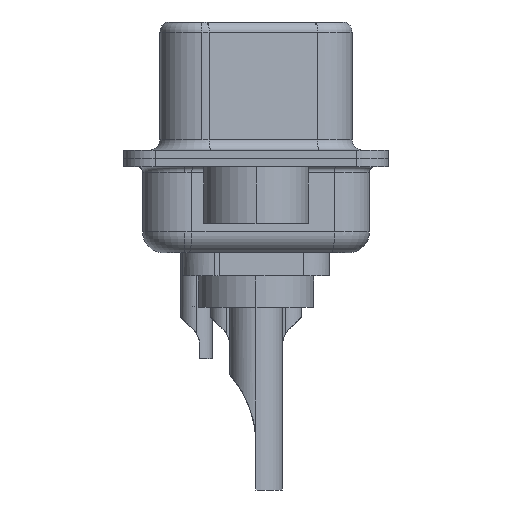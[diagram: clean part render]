
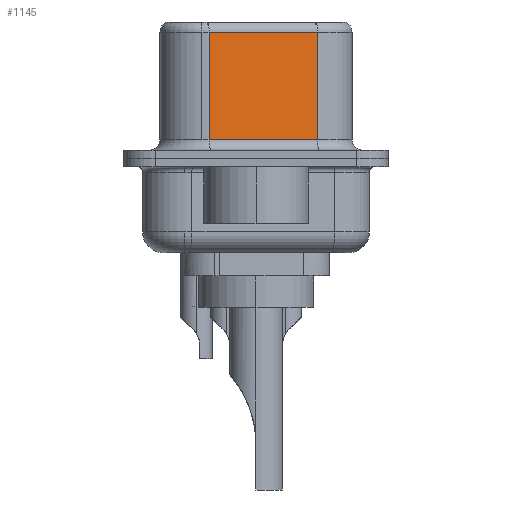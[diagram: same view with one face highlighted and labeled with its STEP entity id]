
A CAD part, left-side view. The second image highlights one B-rep face of the part: STEP entity #1145.
In plain terms, the highlighted planar face has unit normal (-0.985, -0.174, 0).
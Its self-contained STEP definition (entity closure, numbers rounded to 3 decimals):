
#1103 = ORIENTED_EDGE ( 'NONE', *, *, #23241, .T. ) ;
#1145 = ADVANCED_FACE ( 'NONE', ( #22892 ), #13939, .F. ) ;
#1341 = VERTEX_POINT ( 'NONE', #1414 ) ;
#1414 = CARTESIAN_POINT ( 'NONE',  ( 3.67, 2.233, 6.02 ) ) ;
#1542 = CARTESIAN_POINT ( 'NONE',  ( 3.67, 2.233, 0.9 ) ) ;
#1914 = ORIENTED_EDGE ( 'NONE', *, *, #6893, .F. ) ;
#2480 = VECTOR ( 'NONE', #19708, 1000. ) ;
#3179 = CARTESIAN_POINT ( 'NONE',  ( 3.67, 2.233, 6.52 ) ) ;
#4704 = VERTEX_POINT ( 'NONE', #1542 ) ;
#5551 = CARTESIAN_POINT ( 'NONE',  ( 4.58, -2.927, 6.52 ) ) ;
#6531 = ORIENTED_EDGE ( 'NONE', *, *, #21776, .T. ) ;
#6575 = VERTEX_POINT ( 'NONE', #10521 ) ;
#6893 = EDGE_CURVE ( 'NONE', #6575, #12917, #21796, .T. ) ;
#7214 = LINE ( 'NONE', #8791, #2480 ) ;
#7828 = CARTESIAN_POINT ( 'NONE',  ( 4.58, -2.927, 0.9 ) ) ;
#7844 = DIRECTION ( 'NONE',  ( 0., 0., -1. ) ) ;
#8791 = CARTESIAN_POINT ( 'NONE',  ( 4.58, -2.927, 6.02 ) ) ;
#8901 = ORIENTED_EDGE ( 'NONE', *, *, #17003, .T. ) ;
#9419 = VECTOR ( 'NONE', #20563, 1000. ) ;
#10201 = CARTESIAN_POINT ( 'NONE',  ( 4.58, -2.927, 0.9 ) ) ;
#10521 = CARTESIAN_POINT ( 'NONE',  ( 4.58, -2.927, 6.02 ) ) ;
#11525 = DIRECTION ( 'NONE',  ( 0.985, 0.174, 0. ) ) ;
#12054 = VECTOR ( 'NONE', #7844, 1000. ) ;
#12083 = DIRECTION ( 'NONE',  ( 0., 0., -1. ) ) ;
#12336 = VECTOR ( 'NONE', #12083, 1000. ) ;
#12577 = DIRECTION ( 'NONE',  ( -0.174, 0.985, 0. ) ) ;
#12917 = VERTEX_POINT ( 'NONE', #10201 ) ;
#13939 = PLANE ( 'NONE',  #18681 ) ;
#14226 = LINE ( 'NONE', #7828, #9419 ) ;
#17003 = EDGE_CURVE ( 'NONE', #4704, #12917, #14226, .T. ) ;
#18681 = AXIS2_PLACEMENT_3D ( 'NONE', #5551, #11525, #12577 ) ;
#18699 = CARTESIAN_POINT ( 'NONE',  ( 4.58, -2.927, 6.52 ) ) ;
#19708 = DIRECTION ( 'NONE',  ( -0.174, 0.985, 0. ) ) ;
#20563 = DIRECTION ( 'NONE',  ( 0.174, -0.985, 0. ) ) ;
#21082 = EDGE_LOOP ( 'NONE', ( #1914, #1103, #6531, #8901 ) ) ;
#21776 = EDGE_CURVE ( 'NONE', #1341, #4704, #23231, .T. ) ;
#21796 = LINE ( 'NONE', #18699, #12054 ) ;
#22892 = FACE_OUTER_BOUND ( 'NONE', #21082, .T. ) ;
#23231 = LINE ( 'NONE', #3179, #12336 ) ;
#23241 = EDGE_CURVE ( 'NONE', #6575, #1341, #7214, .T. ) ;
